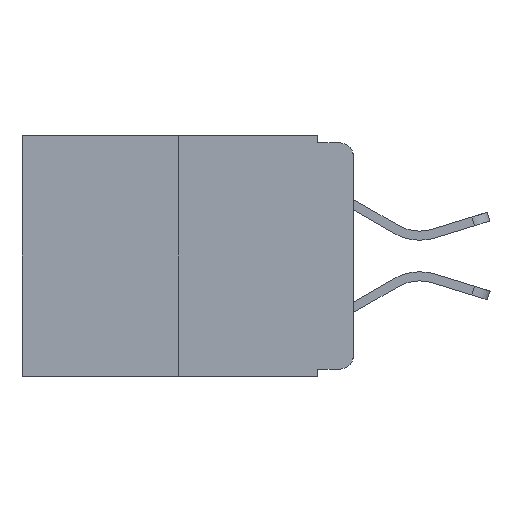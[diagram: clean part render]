
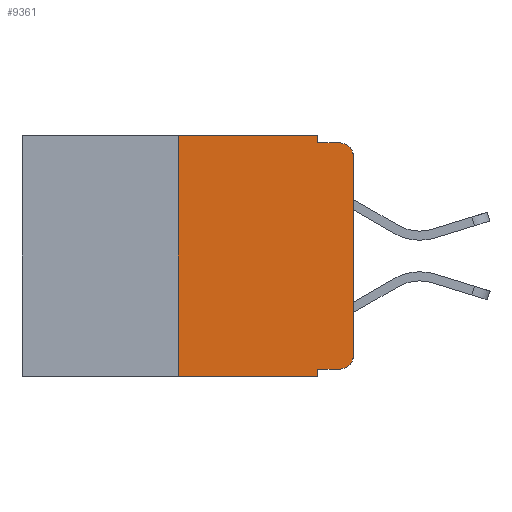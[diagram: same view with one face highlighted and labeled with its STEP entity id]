
A CAD part, left-side view. The second image highlights one B-rep face of the part: STEP entity #9361.
In plain terms, the highlighted planar face has unit normal (-1, 0, 0).
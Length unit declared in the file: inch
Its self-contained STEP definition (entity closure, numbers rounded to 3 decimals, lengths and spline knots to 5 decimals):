
#24 = VERTEX_POINT ( 'NONE', #18544 ) ;
#40 = VERTEX_POINT ( 'NONE', #7069 ) ;
#289 = CARTESIAN_POINT ( 'NONE',  ( 0., 0.02, -0.01 ) ) ;
#641 = EDGE_CURVE ( 'NONE', #2450, #17115, #12314, .T. ) ;
#756 = ORIENTED_EDGE ( 'NONE', *, *, #17188, .F. ) ;
#1193 = DIRECTION ( 'NONE',  ( 0., -1., 0. ) ) ;
#1310 = CARTESIAN_POINT ( 'NONE',  ( 0., 0.051, -0.333 ) ) ;
#1382 = VERTEX_POINT ( 'NONE', #17638 ) ;
#1451 = DIRECTION ( 'NONE',  ( 0., 0., 1. ) ) ;
#1682 = DIRECTION ( 'NONE',  ( 0., -1., 0. ) ) ;
#1689 = LINE ( 'NONE', #11346, #9463 ) ;
#1994 = ORIENTED_EDGE ( 'NONE', *, *, #4014, .T. ) ;
#2450 = VERTEX_POINT ( 'NONE', #12391 ) ;
#2553 = EDGE_CURVE ( 'NONE', #24, #18202, #8042, .T. ) ;
#3153 = VECTOR ( 'NONE', #17857, 39.37008 ) ;
#3421 = VECTOR ( 'NONE', #1682, 39.37008 ) ;
#3650 = PLANE ( 'NONE',  #13426 ) ;
#4014 = EDGE_CURVE ( 'NONE', #17965, #17078, #7611, .T. ) ;
#5131 = VERTEX_POINT ( 'NONE', #8872 ) ;
#5200 = CARTESIAN_POINT ( 'NONE',  ( 0., 0.25, 0. ) ) ;
#5405 = LINE ( 'NONE', #13617, #11872 ) ;
#6144 = VECTOR ( 'NONE', #1193, 39.37008 ) ;
#6375 = CARTESIAN_POINT ( 'NONE',  ( 0., 0.051, 0. ) ) ;
#6658 = CARTESIAN_POINT ( 'NONE',  ( 0., 0.473, 0. ) ) ;
#7069 = CARTESIAN_POINT ( 'NONE',  ( 0., 0.051, -0.343 ) ) ;
#7420 = DIRECTION ( 'NONE',  ( 0., 0., -1. ) ) ;
#7611 = LINE ( 'NONE', #20358, #17342 ) ;
#7648 = LINE ( 'NONE', #10644, #17847 ) ;
#8042 = LINE ( 'NONE', #13124, #3421 ) ;
#8083 = EDGE_CURVE ( 'NONE', #5131, #2450, #13085, .T. ) ;
#8836 = DIRECTION ( 'NONE',  ( 0., -1., 0. ) ) ;
#8872 = CARTESIAN_POINT ( 'NONE',  ( 0., 0.25, -0.343 ) ) ;
#9144 = CARTESIAN_POINT ( 'NONE',  ( 0., 0., -0.313 ) ) ;
#9346 = ORIENTED_EDGE ( 'NONE', *, *, #641, .F. ) ;
#9361 = ADVANCED_FACE ( 'NONE', ( #13300 ), #3650, .F. ) ;
#9400 = EDGE_CURVE ( 'NONE', #17078, #18202, #11763, .T. ) ;
#9463 = VECTOR ( 'NONE', #14811, 39.37008 ) ;
#9978 = EDGE_LOOP ( 'NONE', ( #1994, #11668, #19954, #12505, #9346, #14499, #19823, #756, #17855, #14658 ) ) ;
#10005 = CARTESIAN_POINT ( 'NONE',  ( 0., 0.051, 0. ) ) ;
#10525 = DIRECTION ( 'NONE',  ( -1., 0., 0. ) ) ;
#10584 = CARTESIAN_POINT ( 'NONE',  ( 0., 0.02, -0.03 ) ) ;
#10644 = CARTESIAN_POINT ( 'NONE',  ( 0., 0.473, -0.343 ) ) ;
#10744 = DIRECTION ( 'NONE',  ( 0., -1., 0. ) ) ;
#11346 = CARTESIAN_POINT ( 'NONE',  ( 0., 0.051, 0. ) ) ;
#11517 = DIRECTION ( 'NONE',  ( 0., 0., 1. ) ) ;
#11668 = ORIENTED_EDGE ( 'NONE', *, *, #9400, .T. ) ;
#11763 = CIRCLE ( 'NONE', #19464, 0.02 ) ;
#11837 = DIRECTION ( 'NONE',  ( 0., 0., -1. ) ) ;
#11872 = VECTOR ( 'NONE', #8836, 39.37008 ) ;
#12052 = VECTOR ( 'NONE', #11517, 39.37008 ) ;
#12314 = LINE ( 'NONE', #12411, #6144 ) ;
#12361 = EDGE_CURVE ( 'NONE', #5131, #40, #7648, .T. ) ;
#12391 = CARTESIAN_POINT ( 'NONE',  ( 0., 0.25, 0. ) ) ;
#12411 = CARTESIAN_POINT ( 'NONE',  ( 0., 0.473, 0. ) ) ;
#12505 = ORIENTED_EDGE ( 'NONE', *, *, #17211, .F. ) ;
#13085 = LINE ( 'NONE', #5200, #12052 ) ;
#13124 = CARTESIAN_POINT ( 'NONE',  ( 0., 0.051, -0.01 ) ) ;
#13300 = FACE_OUTER_BOUND ( 'NONE', #9978, .T. ) ;
#13426 = AXIS2_PLACEMENT_3D ( 'NONE', #6658, #19708, #17716 ) ;
#13617 = CARTESIAN_POINT ( 'NONE',  ( 0., 0.051, -0.333 ) ) ;
#13701 = EDGE_CURVE ( 'NONE', #18437, #1382, #5405, .T. ) ;
#13831 = DIRECTION ( 'NONE',  ( -1., 0., 0. ) ) ;
#14499 = ORIENTED_EDGE ( 'NONE', *, *, #8083, .F. ) ;
#14658 = ORIENTED_EDGE ( 'NONE', *, *, #18819, .T. ) ;
#14811 = DIRECTION ( 'NONE',  ( 0., 0., -1. ) ) ;
#15193 = AXIS2_PLACEMENT_3D ( 'NONE', #18489, #10525, #7420 ) ;
#15748 = CARTESIAN_POINT ( 'NONE',  ( 0., 0., -0.03 ) ) ;
#16214 = CIRCLE ( 'NONE', #15193, 0.02 ) ;
#17078 = VERTEX_POINT ( 'NONE', #15748 ) ;
#17115 = VERTEX_POINT ( 'NONE', #6375 ) ;
#17188 = EDGE_CURVE ( 'NONE', #18437, #40, #1689, .T. ) ;
#17211 = EDGE_CURVE ( 'NONE', #17115, #24, #19643, .T. ) ;
#17342 = VECTOR ( 'NONE', #1451, 39.37008 ) ;
#17638 = CARTESIAN_POINT ( 'NONE',  ( 0., 0.02, -0.333 ) ) ;
#17716 = DIRECTION ( 'NONE',  ( 0., 0., -1. ) ) ;
#17847 = VECTOR ( 'NONE', #10744, 39.37008 ) ;
#17855 = ORIENTED_EDGE ( 'NONE', *, *, #13701, .T. ) ;
#17857 = DIRECTION ( 'NONE',  ( 0., 0., -1. ) ) ;
#17965 = VERTEX_POINT ( 'NONE', #9144 ) ;
#18202 = VERTEX_POINT ( 'NONE', #289 ) ;
#18437 = VERTEX_POINT ( 'NONE', #1310 ) ;
#18489 = CARTESIAN_POINT ( 'NONE',  ( 0., 0.02, -0.313 ) ) ;
#18544 = CARTESIAN_POINT ( 'NONE',  ( 0., 0.051, -0.01 ) ) ;
#18819 = EDGE_CURVE ( 'NONE', #1382, #17965, #16214, .T. ) ;
#19464 = AXIS2_PLACEMENT_3D ( 'NONE', #10584, #13831, #11837 ) ;
#19643 = LINE ( 'NONE', #10005, #3153 ) ;
#19708 = DIRECTION ( 'NONE',  ( 1., 0., 0. ) ) ;
#19823 = ORIENTED_EDGE ( 'NONE', *, *, #12361, .T. ) ;
#19954 = ORIENTED_EDGE ( 'NONE', *, *, #2553, .F. ) ;
#20358 = CARTESIAN_POINT ( 'NONE',  ( 0., 0., 0. ) ) ;
